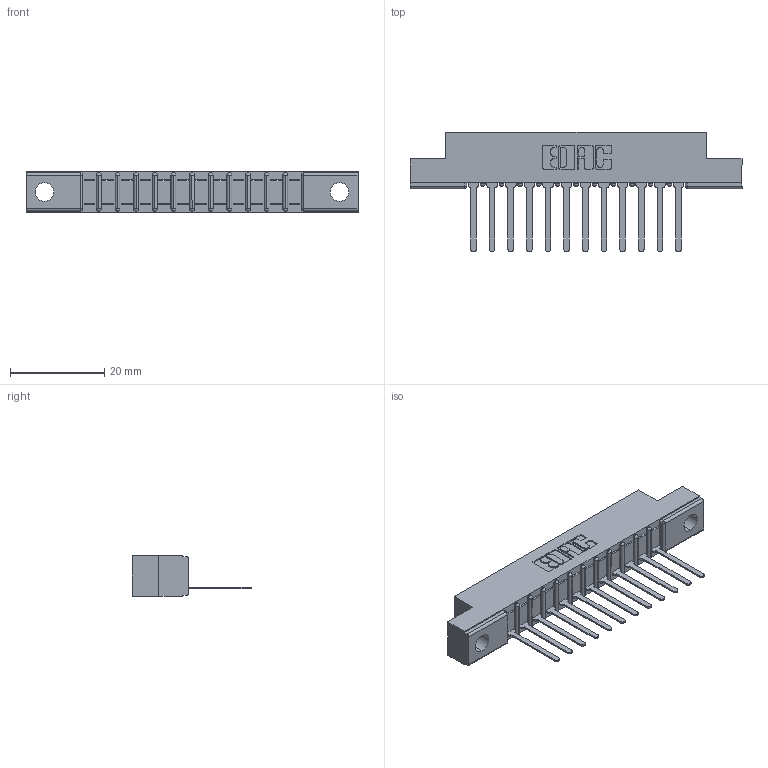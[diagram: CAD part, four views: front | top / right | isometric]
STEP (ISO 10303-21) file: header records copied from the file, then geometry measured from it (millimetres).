
FILE_DESCRIPTION (( 'STEP AP203' ), '1' );
FILE_NAME ('307-012-447-104.STEP', '2020-09-25T11:35:05', ( '' ), ( '' ), 'SwSTEP 2.0', 'SolidWorks 2020', '' );
FILE_SCHEMA (( 'CONFIG_CONTROL_DESIGN' ));
Length unit declared in the file: inch
Products named in the file (3): 307 Part_.156 Dia Mounting Holes; 307-012-447-104; 307-290-001_547
Assembly tree (13 placements, depth 2):
  307-012-447-104
    307 Part_.156 Dia Mounting Holes
    307-290-001_547  x12
Bounding box: 70.56 x 25.43 x 8.71 mm (x, y, z)
Volume: 4401.6 mm3; surface area: 6482.7 mm2
Topology: 13 solids, 13 shells, 817 faces, 2303 edges, 1482 vertices
Faces by surface type: plane 528, cylinder 263, sphere 26
Entity records: 14372 total; most frequent: CARTESIAN_POINT 2414, ORIENTED_EDGE 2398, DIRECTION 2357, EDGE_CURVE 1199, LINE 915, VECTOR 915, VERTEX_POINT 778, AXIS2_PLACEMENT_3D 721
